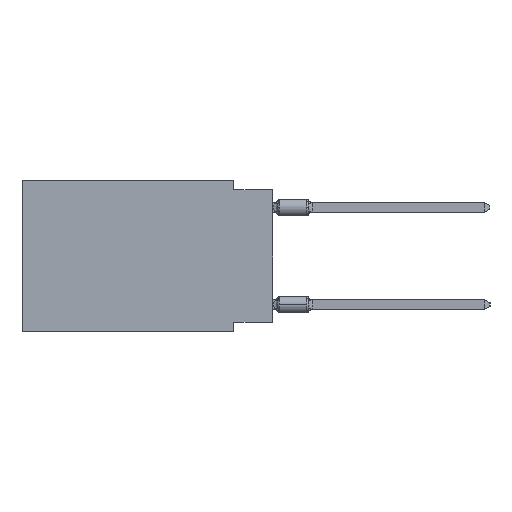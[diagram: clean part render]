
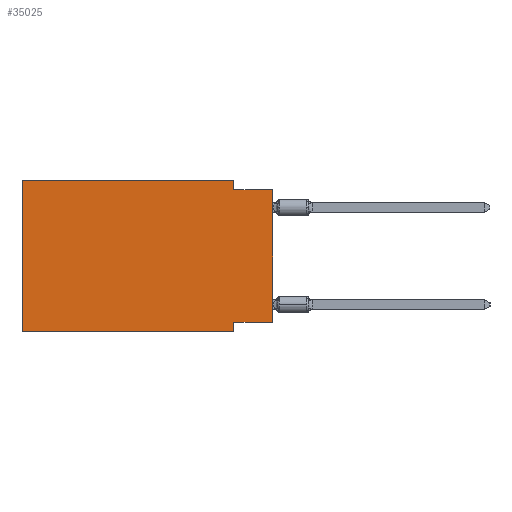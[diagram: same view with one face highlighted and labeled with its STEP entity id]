
A CAD part, left-side view. The second image highlights one B-rep face of the part: STEP entity #35025.
In plain terms, the highlighted planar face has unit normal (-1, 0, 0).
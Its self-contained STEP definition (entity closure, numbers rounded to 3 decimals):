
#401 = LINE ( 'NONE', #33411, #1381 ) ;
#627 = DIRECTION ( 'NONE',  ( 0., 0., -1. ) ) ;
#1381 = VECTOR ( 'NONE', #24165, 1000. ) ;
#1671 = CARTESIAN_POINT ( 'NONE',  ( 0., 0., -9.271 ) ) ;
#2555 = EDGE_CURVE ( 'NONE', #20314, #27712, #401, .T. ) ;
#2729 = VECTOR ( 'NONE', #627, 1000. ) ;
#5663 = VECTOR ( 'NONE', #25430, 1000. ) ;
#6365 = LINE ( 'NONE', #33604, #8204 ) ;
#6418 = CARTESIAN_POINT ( 'NONE',  ( 0., 2.54, -9.906 ) ) ;
#6525 = CARTESIAN_POINT ( 'NONE',  ( 0., 16.383, 0. ) ) ;
#6685 = DIRECTION ( 'NONE',  ( 1., 0., 0. ) ) ;
#7092 = DIRECTION ( 'NONE',  ( 0., -1., 0. ) ) ;
#8088 = CARTESIAN_POINT ( 'NONE',  ( 0., 0., -0.635 ) ) ;
#8204 = VECTOR ( 'NONE', #18170, 1000. ) ;
#8437 = VERTEX_POINT ( 'NONE', #26947 ) ;
#9516 = EDGE_CURVE ( 'NONE', #30793, #20712, #11487, .T. ) ;
#10182 = LINE ( 'NONE', #6525, #30531 ) ;
#11487 = LINE ( 'NONE', #17291, #5663 ) ;
#11571 = DIRECTION ( 'NONE',  ( 0., -1., 0. ) ) ;
#11879 = ORIENTED_EDGE ( 'NONE', *, *, #9516, .F. ) ;
#12789 = CARTESIAN_POINT ( 'NONE',  ( 0., 2.54, 0. ) ) ;
#13656 = CARTESIAN_POINT ( 'NONE',  ( 0., 0., 0. ) ) ;
#13860 = ORIENTED_EDGE ( 'NONE', *, *, #22020, .F. ) ;
#14035 = ORIENTED_EDGE ( 'NONE', *, *, #23006, .F. ) ;
#16073 = LINE ( 'NONE', #12789, #16195 ) ;
#16195 = VECTOR ( 'NONE', #21104, 1000. ) ;
#16348 = ORIENTED_EDGE ( 'NONE', *, *, #34181, .T. ) ;
#16808 = LINE ( 'NONE', #34776, #35108 ) ;
#17290 = EDGE_CURVE ( 'NONE', #22475, #27712, #28359, .T. ) ;
#17291 = CARTESIAN_POINT ( 'NONE',  ( 0., 16.383, 0. ) ) ;
#18170 = DIRECTION ( 'NONE',  ( 0., 1., 0. ) ) ;
#18458 = EDGE_LOOP ( 'NONE', ( #30283, #31426, #14035, #30542, #11879, #16348, #20963, #13860 ) ) ;
#18654 = FACE_OUTER_BOUND ( 'NONE', #18458, .T. ) ;
#18877 = CARTESIAN_POINT ( 'NONE',  ( 0., 2.54, -9.906 ) ) ;
#20043 = CARTESIAN_POINT ( 'NONE',  ( 0., 2.54, -9.271 ) ) ;
#20314 = VERTEX_POINT ( 'NONE', #27468 ) ;
#20712 = VERTEX_POINT ( 'NONE', #24149 ) ;
#20963 = ORIENTED_EDGE ( 'NONE', *, *, #27030, .F. ) ;
#21098 = LINE ( 'NONE', #6418, #2729 ) ;
#21104 = DIRECTION ( 'NONE',  ( 0., 0., -1. ) ) ;
#22020 = EDGE_CURVE ( 'NONE', #22475, #35943, #6365, .T. ) ;
#22475 = VERTEX_POINT ( 'NONE', #1671 ) ;
#23006 = EDGE_CURVE ( 'NONE', #8437, #20314, #16073, .T. ) ;
#23134 = VECTOR ( 'NONE', #25465, 1000. ) ;
#23427 = CARTESIAN_POINT ( 'NONE',  ( 0., 16.383, -9.906 ) ) ;
#24149 = CARTESIAN_POINT ( 'NONE',  ( 0., 16.383, 0. ) ) ;
#24165 = DIRECTION ( 'NONE',  ( 0., -1., 0. ) ) ;
#25237 = CARTESIAN_POINT ( 'NONE',  ( 0., 16.383, 0. ) ) ;
#25326 = AXIS2_PLACEMENT_3D ( 'NONE', #25237, #6685, #27367 ) ;
#25430 = DIRECTION ( 'NONE',  ( 0., 0., 1. ) ) ;
#25465 = DIRECTION ( 'NONE',  ( 0., 0., 1. ) ) ;
#26947 = CARTESIAN_POINT ( 'NONE',  ( 0., 2.54, 0. ) ) ;
#27030 = EDGE_CURVE ( 'NONE', #35943, #27931, #21098, .T. ) ;
#27367 = DIRECTION ( 'NONE',  ( 0., 0., -1. ) ) ;
#27468 = CARTESIAN_POINT ( 'NONE',  ( 0., 2.54, -0.635 ) ) ;
#27712 = VERTEX_POINT ( 'NONE', #8088 ) ;
#27931 = VERTEX_POINT ( 'NONE', #18877 ) ;
#27982 = EDGE_CURVE ( 'NONE', #20712, #8437, #10182, .T. ) ;
#28359 = LINE ( 'NONE', #13656, #23134 ) ;
#30249 = PLANE ( 'NONE',  #25326 ) ;
#30283 = ORIENTED_EDGE ( 'NONE', *, *, #17290, .T. ) ;
#30531 = VECTOR ( 'NONE', #7092, 1000. ) ;
#30542 = ORIENTED_EDGE ( 'NONE', *, *, #27982, .F. ) ;
#30793 = VERTEX_POINT ( 'NONE', #23427 ) ;
#31426 = ORIENTED_EDGE ( 'NONE', *, *, #2555, .F. ) ;
#33411 = CARTESIAN_POINT ( 'NONE',  ( 0., 0., -0.635 ) ) ;
#33604 = CARTESIAN_POINT ( 'NONE',  ( 0., 0., -9.271 ) ) ;
#34181 = EDGE_CURVE ( 'NONE', #30793, #27931, #16808, .T. ) ;
#34776 = CARTESIAN_POINT ( 'NONE',  ( 0., 16.383, -9.906 ) ) ;
#35025 = ADVANCED_FACE ( 'NONE', ( #18654 ), #30249, .F. ) ;
#35108 = VECTOR ( 'NONE', #11571, 1000. ) ;
#35943 = VERTEX_POINT ( 'NONE', #20043 ) ;
